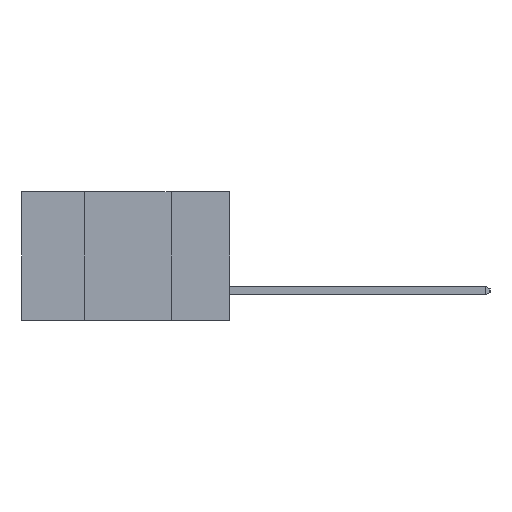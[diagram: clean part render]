
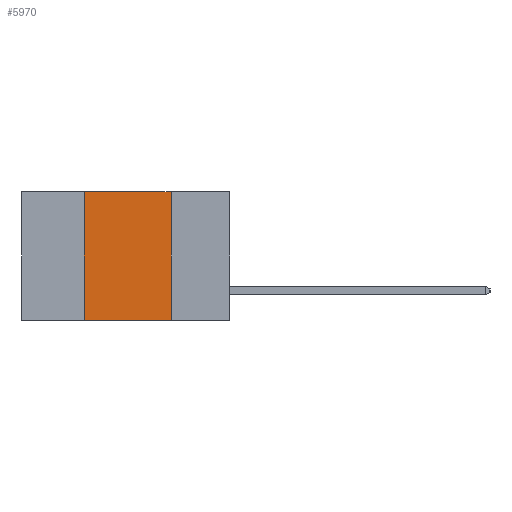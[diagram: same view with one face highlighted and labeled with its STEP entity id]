
A CAD part, left-side view. The second image highlights one B-rep face of the part: STEP entity #5970.
In plain terms, the highlighted planar face has unit normal (-1, 0, 0).
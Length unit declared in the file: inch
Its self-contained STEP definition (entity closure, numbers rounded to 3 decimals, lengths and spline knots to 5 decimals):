
#241 = DIRECTION ( 'NONE',  ( 1., 0., 0. ) ) ;
#1355 = LINE ( 'NONE', #1924, #17586 ) ;
#1616 = VERTEX_POINT ( 'NONE', #11218 ) ;
#1924 = CARTESIAN_POINT ( 'NONE',  ( 0., 0.42, 0. ) ) ;
#2233 = FACE_OUTER_BOUND ( 'NONE', #9935, .T. ) ;
#3285 = DIRECTION ( 'NONE',  ( 0., 0., -1. ) ) ;
#3404 = LINE ( 'NONE', #20173, #13643 ) ;
#3886 = DIRECTION ( 'NONE',  ( 0., 0., 1. ) ) ;
#5970 = ADVANCED_FACE ( 'NONE', ( #2233 ), #12314, .F. ) ;
#6355 = CARTESIAN_POINT ( 'NONE',  ( 0., 0.6, 0. ) ) ;
#6854 = EDGE_CURVE ( 'NONE', #11731, #24447, #24548, .T. ) ;
#7410 = CARTESIAN_POINT ( 'NONE',  ( 0., 0.17, -0.37 ) ) ;
#7869 = DIRECTION ( 'NONE',  ( 0., -1., 0. ) ) ;
#8028 = ORIENTED_EDGE ( 'NONE', *, *, #19624, .T. ) ;
#9935 = EDGE_LOOP ( 'NONE', ( #26091, #13617, #24536, #8028 ) ) ;
#10542 = LINE ( 'NONE', #14092, #15299 ) ;
#11218 = CARTESIAN_POINT ( 'NONE',  ( 0., 0.42, -0.37 ) ) ;
#11731 = VERTEX_POINT ( 'NONE', #13519 ) ;
#12314 = PLANE ( 'NONE',  #17249 ) ;
#13463 = CARTESIAN_POINT ( 'NONE',  ( 0., 0.17, 0. ) ) ;
#13519 = CARTESIAN_POINT ( 'NONE',  ( 0., 0.17, 0. ) ) ;
#13617 = ORIENTED_EDGE ( 'NONE', *, *, #20796, .F. ) ;
#13643 = VECTOR ( 'NONE', #7869, 39.37008 ) ;
#14092 = CARTESIAN_POINT ( 'NONE',  ( 0., 0.6, -0.37 ) ) ;
#14936 = VERTEX_POINT ( 'NONE', #21823 ) ;
#15299 = VECTOR ( 'NONE', #26341, 39.37008 ) ;
#17249 = AXIS2_PLACEMENT_3D ( 'NONE', #6355, #241, #3285 ) ;
#17586 = VECTOR ( 'NONE', #3886, 39.37008 ) ;
#18356 = DIRECTION ( 'NONE',  ( 0., 0., -1. ) ) ;
#18904 = EDGE_CURVE ( 'NONE', #1616, #14936, #1355, .T. ) ;
#19624 = EDGE_CURVE ( 'NONE', #1616, #24447, #10542, .T. ) ;
#20173 = CARTESIAN_POINT ( 'NONE',  ( 0., 0.6, 0. ) ) ;
#20796 = EDGE_CURVE ( 'NONE', #14936, #11731, #3404, .T. ) ;
#21823 = CARTESIAN_POINT ( 'NONE',  ( 0., 0.42, 0. ) ) ;
#23915 = VECTOR ( 'NONE', #18356, 39.37008 ) ;
#24447 = VERTEX_POINT ( 'NONE', #7410 ) ;
#24536 = ORIENTED_EDGE ( 'NONE', *, *, #18904, .F. ) ;
#24548 = LINE ( 'NONE', #13463, #23915 ) ;
#26091 = ORIENTED_EDGE ( 'NONE', *, *, #6854, .F. ) ;
#26341 = DIRECTION ( 'NONE',  ( 0., -1., 0. ) ) ;
